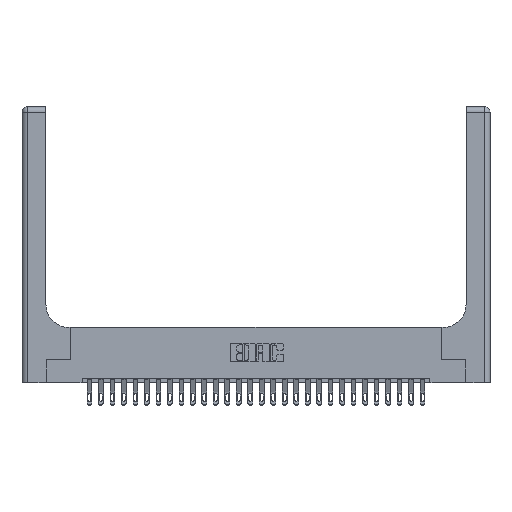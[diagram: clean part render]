
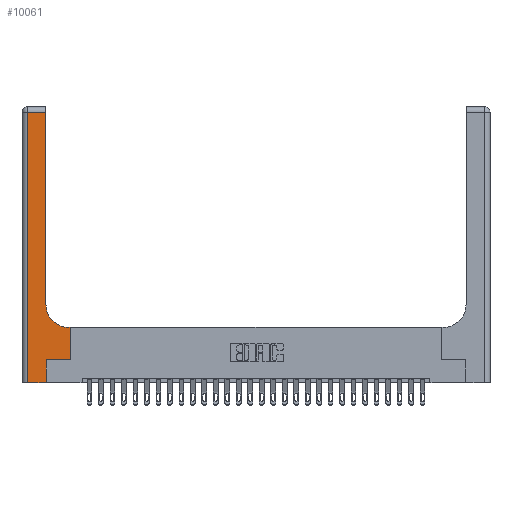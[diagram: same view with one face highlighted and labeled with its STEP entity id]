
A CAD part, top view. The second image highlights one B-rep face of the part: STEP entity #10061.
In plain terms, the highlighted planar face has unit normal (0, 0, 1).
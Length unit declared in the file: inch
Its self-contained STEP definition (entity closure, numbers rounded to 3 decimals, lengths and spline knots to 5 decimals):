
#423 = ORIENTED_EDGE ( 'NONE', *, *, #12849, .T. ) ;
#694 = DIRECTION ( 'NONE',  ( 1., 0., 0. ) ) ;
#975 = LINE ( 'NONE', #9496, #4560 ) ;
#1429 = DIRECTION ( 'NONE',  ( 0., 1., 0. ) ) ;
#1608 = CIRCLE ( 'NONE', #4254, 0.25 ) ;
#3375 = LINE ( 'NONE', #17998, #20392 ) ;
#3418 = CARTESIAN_POINT ( 'NONE',  ( 0.51, 0.6, 0.37 ) ) ;
#3843 = VECTOR ( 'NONE', #21178, 39.37008 ) ;
#4254 = AXIS2_PLACEMENT_3D ( 'NONE', #17464, #7228, #5448 ) ;
#4300 = DIRECTION ( 'NONE',  ( 0., -1., 0. ) ) ;
#4560 = VECTOR ( 'NONE', #4720, 39.37008 ) ;
#4720 = DIRECTION ( 'NONE',  ( -1., 0., 0. ) ) ;
#5448 = DIRECTION ( 'NONE',  ( 1., 0., 0. ) ) ;
#5484 = CARTESIAN_POINT ( 'NONE',  ( 0., 2.94, 0.37 ) ) ;
#5626 = LINE ( 'NONE', #9846, #24814 ) ;
#5682 = ORIENTED_EDGE ( 'NONE', *, *, #12555, .T. ) ;
#5876 = LINE ( 'NONE', #5484, #18170 ) ;
#7051 = CARTESIAN_POINT ( 'NONE',  ( 0.06, 3., 0.37 ) ) ;
#7228 = DIRECTION ( 'NONE',  ( 0., 0., -1. ) ) ;
#7340 = CARTESIAN_POINT ( 'NONE',  ( 0.265, 0., 0.37 ) ) ;
#7394 = FACE_OUTER_BOUND ( 'NONE', #20927, .T. ) ;
#7601 = DIRECTION ( 'NONE',  ( 1., 0., 0. ) ) ;
#7644 = VERTEX_POINT ( 'NONE', #26355 ) ;
#7895 = ORIENTED_EDGE ( 'NONE', *, *, #17950, .T. ) ;
#8034 = VERTEX_POINT ( 'NONE', #17339 ) ;
#8781 = CARTESIAN_POINT ( 'NONE',  ( 0.528, 0.6, 0.37 ) ) ;
#8917 = VECTOR ( 'NONE', #694, 39.37008 ) ;
#9082 = AXIS2_PLACEMENT_3D ( 'NONE', #15668, #20590, #18646 ) ;
#9496 = CARTESIAN_POINT ( 'NONE',  ( 0.26, 0.6, 0.37 ) ) ;
#9846 = CARTESIAN_POINT ( 'NONE',  ( 0.528, 0.25, 0.37 ) ) ;
#9941 = ORIENTED_EDGE ( 'NONE', *, *, #26549, .T. ) ;
#10061 = ADVANCED_FACE ( 'NONE', ( #7394 ), #19813, .F. ) ;
#10122 = EDGE_CURVE ( 'NONE', #20905, #8034, #1608, .T. ) ;
#11128 = VERTEX_POINT ( 'NONE', #24253 ) ;
#11132 = CARTESIAN_POINT ( 'NONE',  ( 0., 0., 0.37 ) ) ;
#11312 = VERTEX_POINT ( 'NONE', #17314 ) ;
#11531 = VERTEX_POINT ( 'NONE', #8781 ) ;
#12136 = DIRECTION ( 'NONE',  ( -1., 0., 0. ) ) ;
#12326 = LINE ( 'NONE', #20719, #20296 ) ;
#12555 = EDGE_CURVE ( 'NONE', #24487, #11312, #5876, .T. ) ;
#12727 = CARTESIAN_POINT ( 'NONE',  ( 0.26, 2.94, 0.37 ) ) ;
#12797 = CARTESIAN_POINT ( 'NONE',  ( 0.265, 0., 0.37 ) ) ;
#12849 = EDGE_CURVE ( 'NONE', #8034, #24487, #3375, .T. ) ;
#13263 = ORIENTED_EDGE ( 'NONE', *, *, #15245, .T. ) ;
#13937 = DIRECTION ( 'NONE',  ( 0., 1., 0. ) ) ;
#14107 = CARTESIAN_POINT ( 'NONE',  ( 0.265, 0.25, 0.37 ) ) ;
#14720 = ORIENTED_EDGE ( 'NONE', *, *, #10122, .T. ) ;
#15245 = EDGE_CURVE ( 'NONE', #11312, #7644, #25816, .T. ) ;
#15668 = CARTESIAN_POINT ( 'NONE',  ( 0., 3., 0.37 ) ) ;
#17314 = CARTESIAN_POINT ( 'NONE',  ( 0.06, 2.94, 0.37 ) ) ;
#17339 = CARTESIAN_POINT ( 'NONE',  ( 0.26, 0.85, 0.37 ) ) ;
#17464 = CARTESIAN_POINT ( 'NONE',  ( 0.51, 0.85, 0.37 ) ) ;
#17950 = EDGE_CURVE ( 'NONE', #19859, #20025, #23207, .T. ) ;
#17998 = CARTESIAN_POINT ( 'NONE',  ( 0.26, 3., 0.37 ) ) ;
#18170 = VECTOR ( 'NONE', #12136, 39.37008 ) ;
#18277 = ORIENTED_EDGE ( 'NONE', *, *, #26400, .T. ) ;
#18442 = VECTOR ( 'NONE', #4300, 39.37008 ) ;
#18646 = DIRECTION ( 'NONE',  ( -1., 0., 0. ) ) ;
#19812 = EDGE_CURVE ( 'NONE', #11531, #20905, #975, .T. ) ;
#19813 = PLANE ( 'NONE',  #9082 ) ;
#19859 = VERTEX_POINT ( 'NONE', #7340 ) ;
#20025 = VERTEX_POINT ( 'NONE', #14107 ) ;
#20212 = ORIENTED_EDGE ( 'NONE', *, *, #23084, .T. ) ;
#20296 = VECTOR ( 'NONE', #7601, 39.37008 ) ;
#20392 = VECTOR ( 'NONE', #1429, 39.37008 ) ;
#20590 = DIRECTION ( 'NONE',  ( 0., 0., -1. ) ) ;
#20719 = CARTESIAN_POINT ( 'NONE',  ( 0.265, 0.25, 0.37 ) ) ;
#20905 = VERTEX_POINT ( 'NONE', #3418 ) ;
#20927 = EDGE_LOOP ( 'NONE', ( #423, #5682, #13263, #18277, #7895, #9941, #20212, #22210, #14720 ) ) ;
#21178 = DIRECTION ( 'NONE',  ( 0., 1., 0. ) ) ;
#21560 = LINE ( 'NONE', #11132, #8917 ) ;
#22210 = ORIENTED_EDGE ( 'NONE', *, *, #19812, .T. ) ;
#23084 = EDGE_CURVE ( 'NONE', #11128, #11531, #5626, .T. ) ;
#23207 = LINE ( 'NONE', #12797, #3843 ) ;
#24253 = CARTESIAN_POINT ( 'NONE',  ( 0.528, 0.25, 0.37 ) ) ;
#24487 = VERTEX_POINT ( 'NONE', #12727 ) ;
#24814 = VECTOR ( 'NONE', #13937, 39.37008 ) ;
#25816 = LINE ( 'NONE', #7051, #18442 ) ;
#26355 = CARTESIAN_POINT ( 'NONE',  ( 0.06, 0., 0.37 ) ) ;
#26400 = EDGE_CURVE ( 'NONE', #7644, #19859, #21560, .T. ) ;
#26549 = EDGE_CURVE ( 'NONE', #20025, #11128, #12326, .T. ) ;
